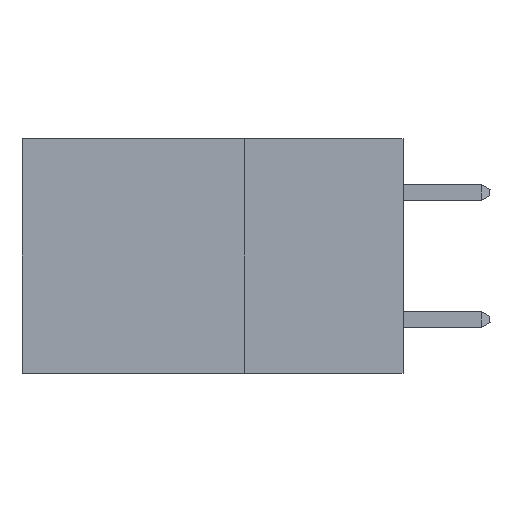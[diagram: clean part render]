
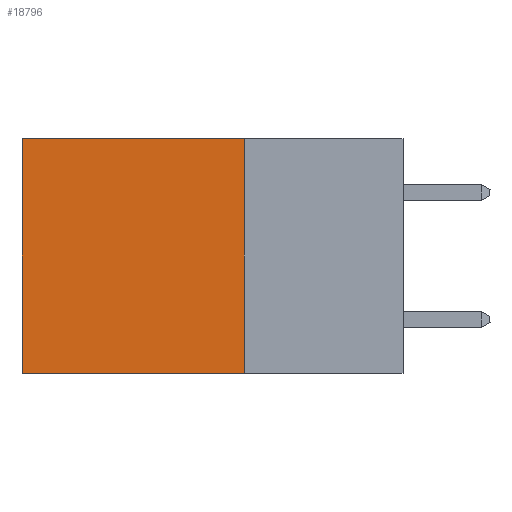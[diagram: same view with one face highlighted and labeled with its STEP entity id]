
A CAD part, left-side view. The second image highlights one B-rep face of the part: STEP entity #18796.
In plain terms, the highlighted planar face has unit normal (-1, 0, 0).
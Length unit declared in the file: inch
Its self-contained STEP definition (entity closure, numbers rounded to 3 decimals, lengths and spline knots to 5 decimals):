
#162 = EDGE_CURVE ( 'NONE', #8247, #3146, #1310, .T. ) ;
#654 = VECTOR ( 'NONE', #10449, 39.37008 ) ;
#1310 = LINE ( 'NONE', #11373, #9455 ) ;
#1600 = EDGE_CURVE ( 'NONE', #11957, #3146, #7994, .T. ) ;
#1675 = EDGE_CURVE ( 'NONE', #3683, #8247, #3098, .T. ) ;
#3098 = LINE ( 'NONE', #17455, #17925 ) ;
#3146 = VERTEX_POINT ( 'NONE', #4525 ) ;
#3461 = ORIENTED_EDGE ( 'NONE', *, *, #1675, .T. ) ;
#3683 = VERTEX_POINT ( 'NONE', #10026 ) ;
#4499 = VECTOR ( 'NONE', #7045, 39.37008 ) ;
#4525 = CARTESIAN_POINT ( 'NONE',  ( 0.2875, 0.6, -0.37 ) ) ;
#4610 = LINE ( 'NONE', #10256, #654 ) ;
#5295 = AXIS2_PLACEMENT_3D ( 'NONE', #12221, #12027, #13643 ) ;
#7045 = DIRECTION ( 'NONE',  ( 0., 1., 0. ) ) ;
#7516 = CARTESIAN_POINT ( 'NONE',  ( 0.2875, 0.6, 0. ) ) ;
#7759 = PLANE ( 'NONE',  #5295 ) ;
#7994 = LINE ( 'NONE', #17390, #4499 ) ;
#8203 = CARTESIAN_POINT ( 'NONE',  ( 0.2875, 0.25, -0.37 ) ) ;
#8247 = VERTEX_POINT ( 'NONE', #7516 ) ;
#8743 = ORIENTED_EDGE ( 'NONE', *, *, #162, .T. ) ;
#8795 = FACE_OUTER_BOUND ( 'NONE', #14889, .T. ) ;
#9455 = VECTOR ( 'NONE', #14344, 39.37008 ) ;
#9931 = ORIENTED_EDGE ( 'NONE', *, *, #1600, .F. ) ;
#10026 = CARTESIAN_POINT ( 'NONE',  ( 0.2875, 0.25, 0. ) ) ;
#10256 = CARTESIAN_POINT ( 'NONE',  ( 0.2875, 0.25, 0. ) ) ;
#10449 = DIRECTION ( 'NONE',  ( 0., 0., -1. ) ) ;
#11373 = CARTESIAN_POINT ( 'NONE',  ( 0.2875, 0.6, 0. ) ) ;
#11957 = VERTEX_POINT ( 'NONE', #8203 ) ;
#12027 = DIRECTION ( 'NONE',  ( 1., 0., 0. ) ) ;
#12221 = CARTESIAN_POINT ( 'NONE',  ( 0.2875, 0.25, 0. ) ) ;
#12446 = ORIENTED_EDGE ( 'NONE', *, *, #13177, .F. ) ;
#13177 = EDGE_CURVE ( 'NONE', #3683, #11957, #4610, .T. ) ;
#13643 = DIRECTION ( 'NONE',  ( 0., 0., -1. ) ) ;
#14344 = DIRECTION ( 'NONE',  ( 0., 0., -1. ) ) ;
#14617 = DIRECTION ( 'NONE',  ( 0., 1., 0. ) ) ;
#14889 = EDGE_LOOP ( 'NONE', ( #8743, #9931, #12446, #3461 ) ) ;
#17390 = CARTESIAN_POINT ( 'NONE',  ( 0.2875, 0.25, -0.37 ) ) ;
#17455 = CARTESIAN_POINT ( 'NONE',  ( 0.2875, 0.25, 0. ) ) ;
#17925 = VECTOR ( 'NONE', #14617, 39.37008 ) ;
#18796 = ADVANCED_FACE ( 'NONE', ( #8795 ), #7759, .F. ) ;
